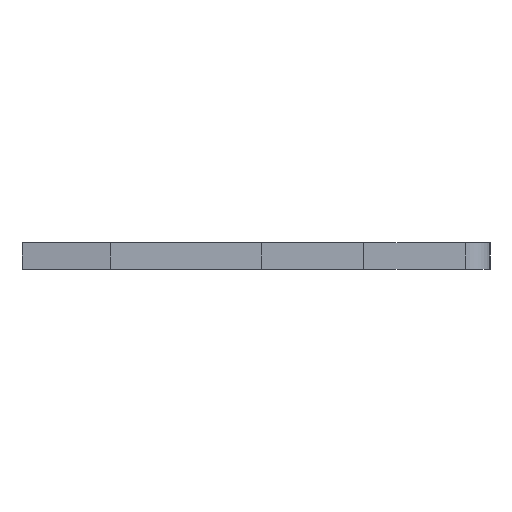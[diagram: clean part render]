
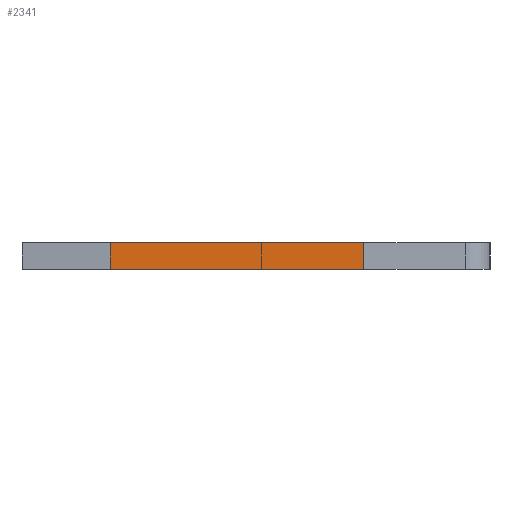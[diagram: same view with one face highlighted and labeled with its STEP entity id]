
A CAD part, left-side view. The second image highlights one B-rep face of the part: STEP entity #2341.
In plain terms, the highlighted face is planar.
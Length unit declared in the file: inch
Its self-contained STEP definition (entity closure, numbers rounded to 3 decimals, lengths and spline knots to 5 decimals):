
#66 = CARTESIAN_POINT ( 'NONE',  ( 0.013, 0.146, -0.0575 ) ) ;
#69 = CARTESIAN_POINT ( 'NONE',  ( 0.013, 0.146, -0.0575 ) ) ;
#76 = PLANE ( 'NONE',  #539 ) ;
#82 = LINE ( 'NONE', #857, #1555 ) ;
#228 = LINE ( 'NONE', #1538, #1523 ) ;
#383 = ORIENTED_EDGE ( 'NONE', *, *, #2067, .T. ) ;
#413 = EDGE_CURVE ( 'NONE', #631, #1437, #1226, .T. ) ;
#419 = LINE ( 'NONE', #1358, #884 ) ;
#424 = ORIENTED_EDGE ( 'NONE', *, *, #633, .F. ) ;
#493 = VERTEX_POINT ( 'NONE', #660 ) ;
#539 = AXIS2_PLACEMENT_3D ( 'NONE', #66, #1052, #1393 ) ;
#611 = DIRECTION ( 'NONE',  ( -1., 0., 0. ) ) ;
#631 = VERTEX_POINT ( 'NONE', #1806 ) ;
#633 = EDGE_CURVE ( 'NONE', #493, #631, #82, .T. ) ;
#660 = CARTESIAN_POINT ( 'NONE',  ( 0.013, -0.099, -0.0575 ) ) ;
#857 = CARTESIAN_POINT ( 'NONE',  ( 0.013, 0.146, -0.0575 ) ) ;
#884 = VECTOR ( 'NONE', #611, 39.37008 ) ;
#936 = DIRECTION ( 'NONE',  ( 0., 1., 0. ) ) ;
#1052 = DIRECTION ( 'NONE',  ( 0., 0., 1. ) ) ;
#1199 = DIRECTION ( 'NONE',  ( -1., 0., 0. ) ) ;
#1226 = LINE ( 'NONE', #69, #1471 ) ;
#1237 = ORIENTED_EDGE ( 'NONE', *, *, #1676, .T. ) ;
#1358 = CARTESIAN_POINT ( 'NONE',  ( 0.013, -0.099, -0.0575 ) ) ;
#1393 = DIRECTION ( 'NONE',  ( 1., 0., 0. ) ) ;
#1421 = CARTESIAN_POINT ( 'NONE',  ( -0.013, -0.099, -0.0575 ) ) ;
#1437 = VERTEX_POINT ( 'NONE', #1529 ) ;
#1455 = DIRECTION ( 'NONE',  ( 0., 1., 0. ) ) ;
#1471 = VECTOR ( 'NONE', #1199, 39.37008 ) ;
#1523 = VECTOR ( 'NONE', #936, 39.37008 ) ;
#1529 = CARTESIAN_POINT ( 'NONE',  ( -0.013, 0.146, -0.0575 ) ) ;
#1538 = CARTESIAN_POINT ( 'NONE',  ( -0.013, 0.146, -0.0575 ) ) ;
#1555 = VECTOR ( 'NONE', #1455, 39.37008 ) ;
#1676 = EDGE_CURVE ( 'NONE', #2307, #1437, #228, .T. ) ;
#1806 = CARTESIAN_POINT ( 'NONE',  ( 0.013, 0.146, -0.0575 ) ) ;
#1856 = ORIENTED_EDGE ( 'NONE', *, *, #413, .F. ) ;
#2024 = FACE_OUTER_BOUND ( 'NONE', #2345, .T. ) ;
#2067 = EDGE_CURVE ( 'NONE', #493, #2307, #419, .T. ) ;
#2307 = VERTEX_POINT ( 'NONE', #1421 ) ;
#2341 = ADVANCED_FACE ( 'NONE', ( #2024 ), #76, .F. ) ;
#2345 = EDGE_LOOP ( 'NONE', ( #1237, #1856, #424, #383 ) ) ;
